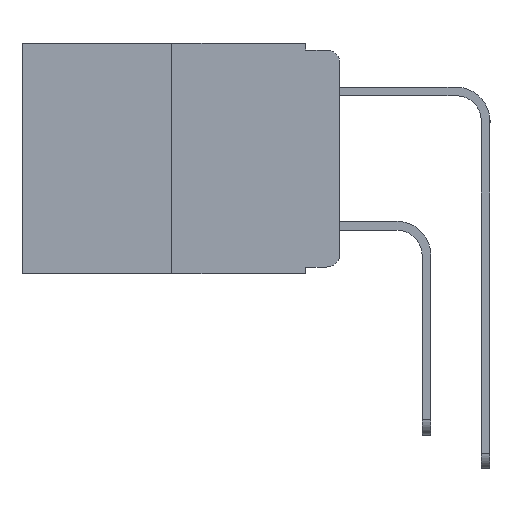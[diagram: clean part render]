
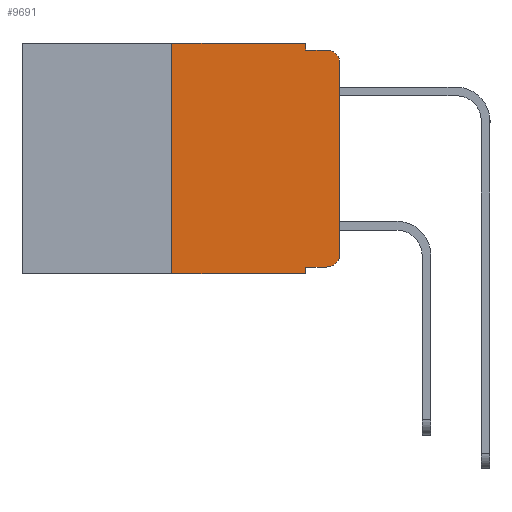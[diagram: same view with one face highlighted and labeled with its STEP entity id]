
A CAD part, left-side view. The second image highlights one B-rep face of the part: STEP entity #9691.
In plain terms, the highlighted planar face has unit normal (-1, 0, 0).
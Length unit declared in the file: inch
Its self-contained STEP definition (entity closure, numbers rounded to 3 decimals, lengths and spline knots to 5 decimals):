
#236 = DIRECTION ( 'NONE',  ( 0., 0., 1. ) ) ;
#338 = VERTEX_POINT ( 'NONE', #11874 ) ;
#425 = DIRECTION ( 'NONE',  ( 0., -1., 0. ) ) ;
#866 = LINE ( 'NONE', #12019, #10465 ) ;
#1290 = ORIENTED_EDGE ( 'NONE', *, *, #11197, .F. ) ;
#1533 = LINE ( 'NONE', #14088, #13884 ) ;
#1956 = VERTEX_POINT ( 'NONE', #3389 ) ;
#2126 = EDGE_CURVE ( 'NONE', #3545, #14573, #15397, .T. ) ;
#2926 = EDGE_CURVE ( 'NONE', #338, #7606, #6697, .T. ) ;
#3199 = EDGE_LOOP ( 'NONE', ( #4384, #7517, #1290, #11027, #8640, #5822, #8983, #12431, #6928, #13872 ) ) ;
#3240 = DIRECTION ( 'NONE',  ( 0., 0., -1. ) ) ;
#3389 = CARTESIAN_POINT ( 'NONE',  ( 0., 0.02, -0.01 ) ) ;
#3545 = VERTEX_POINT ( 'NONE', #13944 ) ;
#3625 = VECTOR ( 'NONE', #15300, 39.37008 ) ;
#3643 = DIRECTION ( 'NONE',  ( 0., 0., -1. ) ) ;
#4091 = EDGE_CURVE ( 'NONE', #14573, #15263, #14327, .T. ) ;
#4215 = CARTESIAN_POINT ( 'NONE',  ( 0., 0., 0. ) ) ;
#4348 = CARTESIAN_POINT ( 'NONE',  ( 0., 0.051, -0.333 ) ) ;
#4384 = ORIENTED_EDGE ( 'NONE', *, *, #4091, .T. ) ;
#4718 = CARTESIAN_POINT ( 'NONE',  ( 0., 0.051, -0.343 ) ) ;
#5043 = CARTESIAN_POINT ( 'NONE',  ( 0., 0., -0.313 ) ) ;
#5216 = VECTOR ( 'NONE', #425, 39.37008 ) ;
#5372 = VERTEX_POINT ( 'NONE', #5744 ) ;
#5744 = CARTESIAN_POINT ( 'NONE',  ( 0., 0.051, -0.01 ) ) ;
#5822 = ORIENTED_EDGE ( 'NONE', *, *, #2926, .F. ) ;
#5915 = CARTESIAN_POINT ( 'NONE',  ( 0., 0., -0.03 ) ) ;
#5917 = EDGE_CURVE ( 'NONE', #7606, #12313, #15131, .T. ) ;
#6236 = LINE ( 'NONE', #4348, #12133 ) ;
#6423 = CIRCLE ( 'NONE', #12540, 0.02 ) ;
#6425 = CARTESIAN_POINT ( 'NONE',  ( 0., 0.051, 0. ) ) ;
#6697 = LINE ( 'NONE', #10395, #3625 ) ;
#6767 = DIRECTION ( 'NONE',  ( -1., 0., 0. ) ) ;
#6862 = DIRECTION ( 'NONE',  ( 0., -1., 0. ) ) ;
#6928 = ORIENTED_EDGE ( 'NONE', *, *, #7054, .T. ) ;
#7054 = EDGE_CURVE ( 'NONE', #12145, #3545, #6236, .T. ) ;
#7258 = DIRECTION ( 'NONE',  ( 0., -1., 0. ) ) ;
#7517 = ORIENTED_EDGE ( 'NONE', *, *, #8817, .T. ) ;
#7569 = VECTOR ( 'NONE', #6862, 39.37008 ) ;
#7606 = VERTEX_POINT ( 'NONE', #10072 ) ;
#8277 = LINE ( 'NONE', #11933, #14387 ) ;
#8640 = ORIENTED_EDGE ( 'NONE', *, *, #5917, .F. ) ;
#8683 = FACE_OUTER_BOUND ( 'NONE', #3199, .T. ) ;
#8817 = EDGE_CURVE ( 'NONE', #15263, #1956, #6423, .T. ) ;
#8877 = AXIS2_PLACEMENT_3D ( 'NONE', #15240, #14979, #14958 ) ;
#8983 = ORIENTED_EDGE ( 'NONE', *, *, #9792, .T. ) ;
#9691 = ADVANCED_FACE ( 'NONE', ( #8683 ), #12550, .F. ) ;
#9792 = EDGE_CURVE ( 'NONE', #338, #12551, #10705, .T. ) ;
#10072 = CARTESIAN_POINT ( 'NONE',  ( 0., 0.25, 0. ) ) ;
#10284 = DIRECTION ( 'NONE',  ( 1., 0., 0. ) ) ;
#10395 = CARTESIAN_POINT ( 'NONE',  ( 0., 0.25, 0. ) ) ;
#10465 = VECTOR ( 'NONE', #10824, 39.37008 ) ;
#10523 = EDGE_CURVE ( 'NONE', #12145, #12551, #1533, .T. ) ;
#10705 = LINE ( 'NONE', #14927, #7569 ) ;
#10824 = DIRECTION ( 'NONE',  ( 0., 0., -1. ) ) ;
#11027 = ORIENTED_EDGE ( 'NONE', *, *, #11953, .F. ) ;
#11197 = EDGE_CURVE ( 'NONE', #5372, #1956, #8277, .T. ) ;
#11321 = VECTOR ( 'NONE', #236, 39.37008 ) ;
#11874 = CARTESIAN_POINT ( 'NONE',  ( 0., 0.25, -0.343 ) ) ;
#11933 = CARTESIAN_POINT ( 'NONE',  ( 0., 0.051, -0.01 ) ) ;
#11953 = EDGE_CURVE ( 'NONE', #12313, #5372, #866, .T. ) ;
#12019 = CARTESIAN_POINT ( 'NONE',  ( 0., 0.051, 0. ) ) ;
#12133 = VECTOR ( 'NONE', #14753, 39.37008 ) ;
#12145 = VERTEX_POINT ( 'NONE', #12205 ) ;
#12205 = CARTESIAN_POINT ( 'NONE',  ( 0., 0.051, -0.333 ) ) ;
#12313 = VERTEX_POINT ( 'NONE', #6425 ) ;
#12431 = ORIENTED_EDGE ( 'NONE', *, *, #10523, .F. ) ;
#12540 = AXIS2_PLACEMENT_3D ( 'NONE', #13777, #6767, #14850 ) ;
#12543 = CARTESIAN_POINT ( 'NONE',  ( 0., 0.473, 0. ) ) ;
#12550 = PLANE ( 'NONE',  #13994 ) ;
#12551 = VERTEX_POINT ( 'NONE', #4718 ) ;
#13703 = CARTESIAN_POINT ( 'NONE',  ( 0., 0.473, 0. ) ) ;
#13777 = CARTESIAN_POINT ( 'NONE',  ( 0., 0.02, -0.03 ) ) ;
#13872 = ORIENTED_EDGE ( 'NONE', *, *, #2126, .T. ) ;
#13884 = VECTOR ( 'NONE', #3643, 39.37008 ) ;
#13944 = CARTESIAN_POINT ( 'NONE',  ( 0., 0.02, -0.333 ) ) ;
#13994 = AXIS2_PLACEMENT_3D ( 'NONE', #13703, #10284, #3240 ) ;
#14088 = CARTESIAN_POINT ( 'NONE',  ( 0., 0.051, 0. ) ) ;
#14327 = LINE ( 'NONE', #4215, #11321 ) ;
#14387 = VECTOR ( 'NONE', #7258, 39.37008 ) ;
#14573 = VERTEX_POINT ( 'NONE', #5043 ) ;
#14753 = DIRECTION ( 'NONE',  ( 0., -1., 0. ) ) ;
#14850 = DIRECTION ( 'NONE',  ( 0., 0., -1. ) ) ;
#14927 = CARTESIAN_POINT ( 'NONE',  ( 0., 0.473, -0.343 ) ) ;
#14958 = DIRECTION ( 'NONE',  ( 0., 0., -1. ) ) ;
#14979 = DIRECTION ( 'NONE',  ( -1., 0., 0. ) ) ;
#15131 = LINE ( 'NONE', #12543, #5216 ) ;
#15240 = CARTESIAN_POINT ( 'NONE',  ( 0., 0.02, -0.313 ) ) ;
#15263 = VERTEX_POINT ( 'NONE', #5915 ) ;
#15300 = DIRECTION ( 'NONE',  ( 0., 0., 1. ) ) ;
#15397 = CIRCLE ( 'NONE', #8877, 0.02 ) ;
